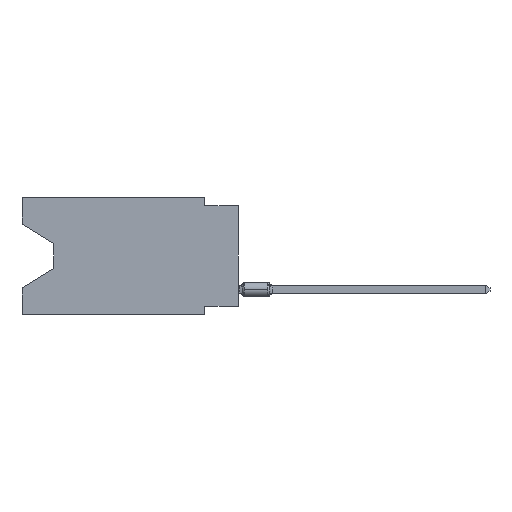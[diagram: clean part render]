
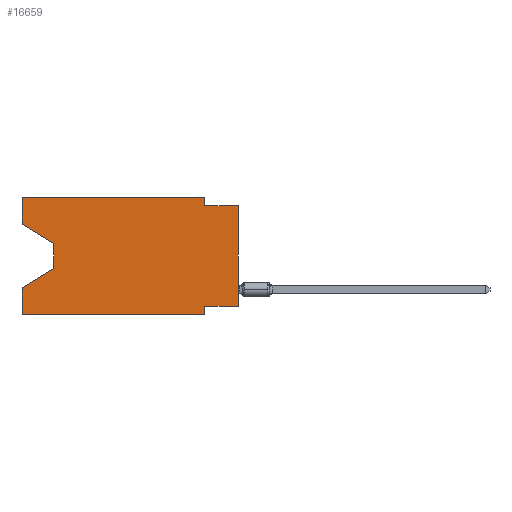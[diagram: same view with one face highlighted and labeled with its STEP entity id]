
A CAD part, left-side view. The second image highlights one B-rep face of the part: STEP entity #16659.
In plain terms, the highlighted planar face has unit normal (-1, 0, 0).
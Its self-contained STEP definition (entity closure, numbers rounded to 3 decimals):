
#810 = ORIENTED_EDGE ( 'NONE', *, *, #29448, .T. ) ;
#1165 = VECTOR ( 'NONE', #7805, 1000. ) ;
#1429 = DIRECTION ( 'NONE',  ( 1., 0., 0. ) ) ;
#1439 = CARTESIAN_POINT ( 'NONE',  ( 0., 16.383, 0. ) ) ;
#1744 = DIRECTION ( 'NONE',  ( 0., 0., -1. ) ) ;
#2085 = ORIENTED_EDGE ( 'NONE', *, *, #17260, .T. ) ;
#2482 = VECTOR ( 'NONE', #29103, 1000. ) ;
#2610 = DIRECTION ( 'NONE',  ( 0., 0., 1. ) ) ;
#2650 = LINE ( 'NONE', #10324, #1165 ) ;
#2667 = VECTOR ( 'NONE', #2610, 1000. ) ;
#3003 = CARTESIAN_POINT ( 'NONE',  ( 0., 13.97, -5.385 ) ) ;
#3389 = DIRECTION ( 'NONE',  ( 0., 0., -1. ) ) ;
#3564 = VECTOR ( 'NONE', #12580, 1000. ) ;
#3786 = VERTEX_POINT ( 'NONE', #31419 ) ;
#4014 = EDGE_CURVE ( 'NONE', #20767, #3786, #16330, .T. ) ;
#4091 = VECTOR ( 'NONE', #17580, 1000. ) ;
#4341 = CARTESIAN_POINT ( 'NONE',  ( 0., 16.383, 0. ) ) ;
#4485 = DIRECTION ( 'NONE',  ( 0., 0., 1. ) ) ;
#4801 = CARTESIAN_POINT ( 'NONE',  ( 0., 0., -0.635 ) ) ;
#5029 = CARTESIAN_POINT ( 'NONE',  ( 0., 16.383, 0. ) ) ;
#5218 = ORIENTED_EDGE ( 'NONE', *, *, #5997, .F. ) ;
#5774 = VECTOR ( 'NONE', #19324, 1000. ) ;
#5870 = VECTOR ( 'NONE', #25673, 1000. ) ;
#5997 = EDGE_CURVE ( 'NONE', #27079, #31736, #18439, .T. ) ;
#6441 = VERTEX_POINT ( 'NONE', #23735 ) ;
#6870 = CARTESIAN_POINT ( 'NONE',  ( 0., 16.383, -8.89 ) ) ;
#7805 = DIRECTION ( 'NONE',  ( 0., 0., 1. ) ) ;
#8590 = DIRECTION ( 'NONE',  ( 0., -0.855, -0.519 ) ) ;
#8632 = FACE_OUTER_BOUND ( 'NONE', #15981, .T. ) ;
#8742 = CARTESIAN_POINT ( 'NONE',  ( 0., 16.383, -2.038 ) ) ;
#8950 = PLANE ( 'NONE',  #28772 ) ;
#9119 = LINE ( 'NONE', #9620, #5774 ) ;
#9620 = CARTESIAN_POINT ( 'NONE',  ( 0., 0., -0.635 ) ) ;
#9809 = VERTEX_POINT ( 'NONE', #23201 ) ;
#10153 = VERTEX_POINT ( 'NONE', #14990 ) ;
#10324 = CARTESIAN_POINT ( 'NONE',  ( 0., 16.383, 0. ) ) ;
#10528 = VECTOR ( 'NONE', #3389, 1000. ) ;
#11465 = CARTESIAN_POINT ( 'NONE',  ( 0., 0., -8.255 ) ) ;
#11605 = VERTEX_POINT ( 'NONE', #19489 ) ;
#11678 = VERTEX_POINT ( 'NONE', #1439 ) ;
#11682 = CARTESIAN_POINT ( 'NONE',  ( 0., 13.97, -3.505 ) ) ;
#11712 = ORIENTED_EDGE ( 'NONE', *, *, #31231, .F. ) ;
#12131 = VECTOR ( 'NONE', #1744, 1000. ) ;
#12580 = DIRECTION ( 'NONE',  ( 0., 0., -1. ) ) ;
#12749 = ORIENTED_EDGE ( 'NONE', *, *, #18807, .F. ) ;
#13415 = EDGE_CURVE ( 'NONE', #6441, #11678, #2650, .T. ) ;
#14100 = LINE ( 'NONE', #19455, #12131 ) ;
#14937 = LINE ( 'NONE', #19946, #3564 ) ;
#14990 = CARTESIAN_POINT ( 'NONE',  ( 0., 16.383, -6.852 ) ) ;
#15603 = EDGE_CURVE ( 'NONE', #3786, #9809, #14937, .T. ) ;
#15981 = EDGE_LOOP ( 'NONE', ( #2085, #19701, #26281, #11712, #810, #20908, #17107, #18206, #12749, #5218, #30903, #28304 ) ) ;
#16128 = VERTEX_POINT ( 'NONE', #3003 ) ;
#16330 = LINE ( 'NONE', #11465, #32735 ) ;
#16659 = ADVANCED_FACE ( 'NONE', ( #8632 ), #8950, .F. ) ;
#16974 = VECTOR ( 'NONE', #4485, 1000. ) ;
#17035 = LINE ( 'NONE', #4341, #16974 ) ;
#17107 = ORIENTED_EDGE ( 'NONE', *, *, #4014, .F. ) ;
#17260 = EDGE_CURVE ( 'NONE', #6441, #29832, #28629, .T. ) ;
#17580 = DIRECTION ( 'NONE',  ( 0., -1., 0. ) ) ;
#18206 = ORIENTED_EDGE ( 'NONE', *, *, #27479, .T. ) ;
#18439 = LINE ( 'NONE', #23286, #10528 ) ;
#18807 = EDGE_CURVE ( 'NONE', #31736, #26482, #9119, .T. ) ;
#19324 = DIRECTION ( 'NONE',  ( 0., -1., 0. ) ) ;
#19455 = CARTESIAN_POINT ( 'NONE',  ( 0., 13.97, -3.505 ) ) ;
#19489 = CARTESIAN_POINT ( 'NONE',  ( 0., 16.383, -8.89 ) ) ;
#19701 = ORIENTED_EDGE ( 'NONE', *, *, #30772, .T. ) ;
#19946 = CARTESIAN_POINT ( 'NONE',  ( 0., 2.54, -8.89 ) ) ;
#20172 = CARTESIAN_POINT ( 'NONE',  ( 0., 2.54, -0.635 ) ) ;
#20190 = CARTESIAN_POINT ( 'NONE',  ( 0., 0., -8.255 ) ) ;
#20767 = VERTEX_POINT ( 'NONE', #20190 ) ;
#20908 = ORIENTED_EDGE ( 'NONE', *, *, #15603, .F. ) ;
#21651 = CARTESIAN_POINT ( 'NONE',  ( 0., 16.383, 0. ) ) ;
#23201 = CARTESIAN_POINT ( 'NONE',  ( 0., 2.54, -8.89 ) ) ;
#23286 = CARTESIAN_POINT ( 'NONE',  ( 0., 2.54, 0. ) ) ;
#23735 = CARTESIAN_POINT ( 'NONE',  ( 0., 16.383, -2.038 ) ) ;
#25002 = LINE ( 'NONE', #25331, #2667 ) ;
#25096 = CARTESIAN_POINT ( 'NONE',  ( 0., 2.54, 0. ) ) ;
#25331 = CARTESIAN_POINT ( 'NONE',  ( 0., 0., 0. ) ) ;
#25599 = LINE ( 'NONE', #5029, #4091 ) ;
#25673 = DIRECTION ( 'NONE',  ( 0., 0.855, -0.519 ) ) ;
#26281 = ORIENTED_EDGE ( 'NONE', *, *, #27571, .T. ) ;
#26482 = VERTEX_POINT ( 'NONE', #4801 ) ;
#26687 = DIRECTION ( 'NONE',  ( 0., 0., -1. ) ) ;
#27079 = VERTEX_POINT ( 'NONE', #25096 ) ;
#27479 = EDGE_CURVE ( 'NONE', #20767, #26482, #25002, .T. ) ;
#27571 = EDGE_CURVE ( 'NONE', #16128, #10153, #27676, .T. ) ;
#27676 = LINE ( 'NONE', #28168, #5870 ) ;
#28168 = CARTESIAN_POINT ( 'NONE',  ( 0., 13.97, -5.385 ) ) ;
#28304 = ORIENTED_EDGE ( 'NONE', *, *, #13415, .F. ) ;
#28629 = LINE ( 'NONE', #8742, #30961 ) ;
#28772 = AXIS2_PLACEMENT_3D ( 'NONE', #21651, #1429, #26687 ) ;
#29103 = DIRECTION ( 'NONE',  ( 0., -1., 0. ) ) ;
#29448 = EDGE_CURVE ( 'NONE', #11605, #9809, #29766, .T. ) ;
#29552 = EDGE_CURVE ( 'NONE', #11678, #27079, #25599, .T. ) ;
#29766 = LINE ( 'NONE', #6870, #2482 ) ;
#29832 = VERTEX_POINT ( 'NONE', #11682 ) ;
#30772 = EDGE_CURVE ( 'NONE', #29832, #16128, #14100, .T. ) ;
#30903 = ORIENTED_EDGE ( 'NONE', *, *, #29552, .F. ) ;
#30961 = VECTOR ( 'NONE', #8590, 1000. ) ;
#31231 = EDGE_CURVE ( 'NONE', #11605, #10153, #17035, .T. ) ;
#31419 = CARTESIAN_POINT ( 'NONE',  ( 0., 2.54, -8.255 ) ) ;
#31736 = VERTEX_POINT ( 'NONE', #20172 ) ;
#31853 = DIRECTION ( 'NONE',  ( 0., 1., 0. ) ) ;
#32735 = VECTOR ( 'NONE', #31853, 1000. ) ;
